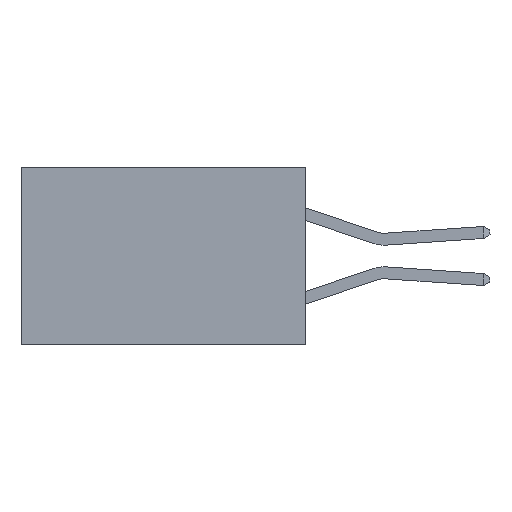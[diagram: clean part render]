
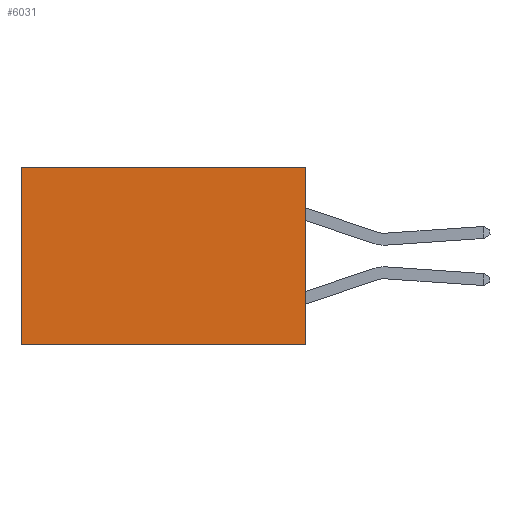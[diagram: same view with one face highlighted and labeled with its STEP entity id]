
A CAD part, left-side view. The second image highlights one B-rep face of the part: STEP entity #6031.
In plain terms, the highlighted planar face has unit normal (-1, 0, 0).
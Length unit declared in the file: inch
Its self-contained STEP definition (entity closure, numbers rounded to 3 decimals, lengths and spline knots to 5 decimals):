
#670 = EDGE_CURVE ( 'NONE', #3550, #5194, #9808, .T. ) ;
#774 = CARTESIAN_POINT ( 'NONE',  ( 0.277, 0.59, 0. ) ) ;
#911 = VECTOR ( 'NONE', #8258, 39.37008 ) ;
#1188 = CARTESIAN_POINT ( 'NONE',  ( 0.277, 0.59, -0.37 ) ) ;
#1273 = VECTOR ( 'NONE', #6607, 39.37008 ) ;
#1573 = CARTESIAN_POINT ( 'NONE',  ( 0.277, 0., -0.37 ) ) ;
#1775 = ORIENTED_EDGE ( 'NONE', *, *, #670, .T. ) ;
#2267 = VERTEX_POINT ( 'NONE', #1188 ) ;
#2269 = LINE ( 'NONE', #3682, #4266 ) ;
#2770 = EDGE_CURVE ( 'NONE', #3550, #5456, #3538, .T. ) ;
#3019 = CARTESIAN_POINT ( 'NONE',  ( 0.277, 0., 0. ) ) ;
#3318 = FACE_OUTER_BOUND ( 'NONE', #10103, .T. ) ;
#3538 = LINE ( 'NONE', #6342, #1273 ) ;
#3550 = VERTEX_POINT ( 'NONE', #3019 ) ;
#3609 = DIRECTION ( 'NONE',  ( 0., 0., -1. ) ) ;
#3682 = CARTESIAN_POINT ( 'NONE',  ( 0.277, 0.59, -0.37 ) ) ;
#4266 = VECTOR ( 'NONE', #3609, 39.37008 ) ;
#5107 = DIRECTION ( 'NONE',  ( 0., 0., -1. ) ) ;
#5123 = DIRECTION ( 'NONE',  ( 1., 0., 0. ) ) ;
#5182 = CARTESIAN_POINT ( 'NONE',  ( 0.277, 0., -0.37 ) ) ;
#5194 = VERTEX_POINT ( 'NONE', #774 ) ;
#5213 = PLANE ( 'NONE',  #9222 ) ;
#5456 = VERTEX_POINT ( 'NONE', #1573 ) ;
#6031 = ADVANCED_FACE ( 'NONE', ( #3318 ), #5213, .F. ) ;
#6342 = CARTESIAN_POINT ( 'NONE',  ( 0.277, 0., -0.37 ) ) ;
#6607 = DIRECTION ( 'NONE',  ( 0., 0., -1. ) ) ;
#7228 = CARTESIAN_POINT ( 'NONE',  ( 0.277, 0., -0.37 ) ) ;
#7405 = ORIENTED_EDGE ( 'NONE', *, *, #7889, .F. ) ;
#7498 = DIRECTION ( 'NONE',  ( 0., 1., 0. ) ) ;
#7643 = CARTESIAN_POINT ( 'NONE',  ( 0.277, 0., 0. ) ) ;
#7887 = VECTOR ( 'NONE', #7498, 39.37008 ) ;
#7889 = EDGE_CURVE ( 'NONE', #5456, #2267, #10034, .T. ) ;
#8258 = DIRECTION ( 'NONE',  ( 0., 1., 0. ) ) ;
#8444 = ORIENTED_EDGE ( 'NONE', *, *, #8697, .T. ) ;
#8697 = EDGE_CURVE ( 'NONE', #5194, #2267, #2269, .T. ) ;
#8944 = ORIENTED_EDGE ( 'NONE', *, *, #2770, .F. ) ;
#9222 = AXIS2_PLACEMENT_3D ( 'NONE', #5182, #5123, #5107 ) ;
#9808 = LINE ( 'NONE', #7643, #911 ) ;
#10034 = LINE ( 'NONE', #7228, #7887 ) ;
#10103 = EDGE_LOOP ( 'NONE', ( #8444, #7405, #8944, #1775 ) ) ;
